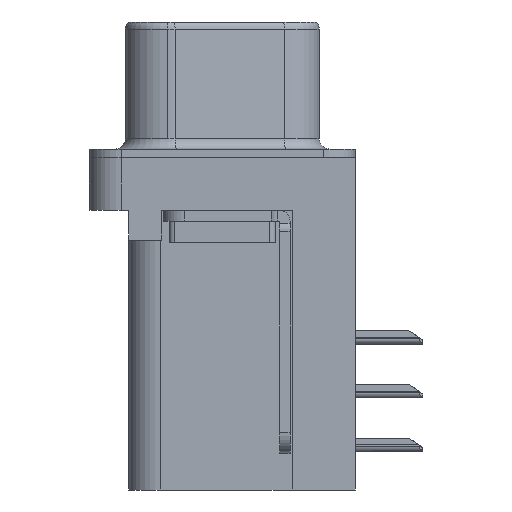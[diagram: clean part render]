
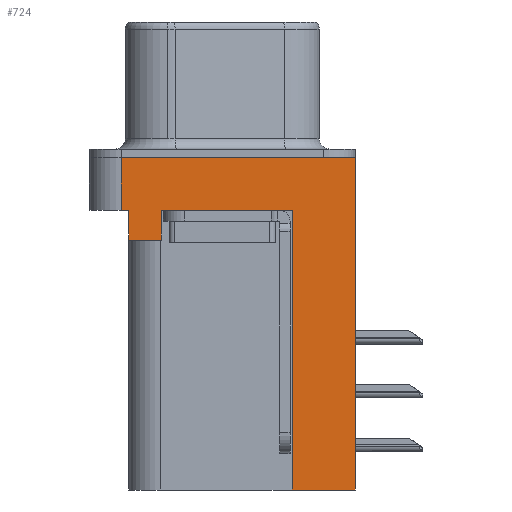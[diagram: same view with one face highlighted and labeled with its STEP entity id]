
A CAD part, left-side view. The second image highlights one B-rep face of the part: STEP entity #724.
In plain terms, the highlighted planar face has unit normal (-1, 0, 0).
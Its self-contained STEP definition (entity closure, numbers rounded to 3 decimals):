
#7 = LINE ( 'NONE', #4996, #25877 ) ;
#96 = VECTOR ( 'NONE', #20133, 1000. ) ;
#724 = ADVANCED_FACE ( 'NONE', ( #19348 ), #10806, .T. ) ;
#2074 = LINE ( 'NONE', #29223, #28957 ) ;
#3903 = CARTESIAN_POINT ( 'NONE',  ( -2.91, -6.275, 0. ) ) ;
#4432 = ORIENTED_EDGE ( 'NONE', *, *, #19202, .F. ) ;
#4996 = CARTESIAN_POINT ( 'NONE',  ( -2.91, -6.275, -2.5 ) ) ;
#5972 = EDGE_LOOP ( 'NONE', ( #6195, #30867, #8219, #24992, #11802, #33199, #10600, #34072, #4432, #23810 ) ) ;
#6113 = CARTESIAN_POINT ( 'NONE',  ( -2.91, -6.275, -2.5 ) ) ;
#6195 = ORIENTED_EDGE ( 'NONE', *, *, #15542, .F. ) ;
#6277 = LINE ( 'NONE', #28604, #28622 ) ;
#6493 = EDGE_CURVE ( 'NONE', #25158, #12339, #13691, .T. ) ;
#7218 = DIRECTION ( 'NONE',  ( 0., 1., 0. ) ) ;
#7662 = DIRECTION ( 'NONE',  ( 0., 0., 1. ) ) ;
#8219 = ORIENTED_EDGE ( 'NONE', *, *, #26451, .T. ) ;
#8778 = DIRECTION ( 'NONE',  ( 0., -1., 0. ) ) ;
#9291 = VERTEX_POINT ( 'NONE', #13595 ) ;
#9411 = CARTESIAN_POINT ( 'NONE',  ( -2.91, -3.295, -15.7 ) ) ;
#10600 = ORIENTED_EDGE ( 'NONE', *, *, #6493, .T. ) ;
#10667 = DIRECTION ( 'NONE',  ( 0., 0., 1. ) ) ;
#10806 = PLANE ( 'NONE',  #26622 ) ;
#10935 = VECTOR ( 'NONE', #10667, 1000. ) ;
#11802 = ORIENTED_EDGE ( 'NONE', *, *, #16735, .F. ) ;
#12339 = VERTEX_POINT ( 'NONE', #22976 ) ;
#12452 = DIRECTION ( 'NONE',  ( 0., 0., 1. ) ) ;
#12564 = DIRECTION ( 'NONE',  ( 0., 0., 1. ) ) ;
#12599 = CARTESIAN_POINT ( 'NONE',  ( -2.91, 2.895, -2.5 ) ) ;
#12738 = VERTEX_POINT ( 'NONE', #26831 ) ;
#13177 = VERTEX_POINT ( 'NONE', #34198 ) ;
#13595 = CARTESIAN_POINT ( 'NONE',  ( -2.91, 4.425, -2.5 ) ) ;
#13691 = LINE ( 'NONE', #6113, #27205 ) ;
#13717 = LINE ( 'NONE', #17897, #27230 ) ;
#13743 = CARTESIAN_POINT ( 'NONE',  ( -2.91, 4.775, -2.5 ) ) ;
#14590 = EDGE_CURVE ( 'NONE', #31923, #9291, #15024, .T. ) ;
#15024 = LINE ( 'NONE', #17603, #96 ) ;
#15542 = EDGE_CURVE ( 'NONE', #12738, #22639, #13717, .T. ) ;
#16201 = EDGE_CURVE ( 'NONE', #22479, #12738, #24565, .T. ) ;
#16735 = EDGE_CURVE ( 'NONE', #30396, #31923, #17400, .T. ) ;
#17128 = VECTOR ( 'NONE', #12452, 1000. ) ;
#17400 = LINE ( 'NONE', #25851, #31253 ) ;
#17603 = CARTESIAN_POINT ( 'NONE',  ( -2.91, 4.425, -3.9 ) ) ;
#17775 = CARTESIAN_POINT ( 'NONE',  ( -2.91, -3.295, -15.7 ) ) ;
#17841 = EDGE_CURVE ( 'NONE', #30396, #25158, #17972, .T. ) ;
#17897 = CARTESIAN_POINT ( 'NONE',  ( -2.91, -6.275, 0. ) ) ;
#17972 = LINE ( 'NONE', #29623, #10935 ) ;
#18573 = EDGE_CURVE ( 'NONE', #29237, #12339, #31879, .T. ) ;
#19202 = EDGE_CURVE ( 'NONE', #13177, #29237, #6277, .T. ) ;
#19348 = FACE_OUTER_BOUND ( 'NONE', #5972, .T. ) ;
#20133 = DIRECTION ( 'NONE',  ( 0., 0., 1. ) ) ;
#20556 = EDGE_CURVE ( 'NONE', #13177, #22639, #7, .T. ) ;
#20946 = DIRECTION ( 'NONE',  ( 0., 0., 1. ) ) ;
#21137 = CARTESIAN_POINT ( 'NONE',  ( -2.91, 4.425, -3.9 ) ) ;
#22404 = CARTESIAN_POINT ( 'NONE',  ( -2.91, 2.895, -3.9 ) ) ;
#22479 = VERTEX_POINT ( 'NONE', #13743 ) ;
#22639 = VERTEX_POINT ( 'NONE', #3903 ) ;
#22976 = CARTESIAN_POINT ( 'NONE',  ( -2.91, -3.295, -2.5 ) ) ;
#23595 = DIRECTION ( 'NONE',  ( 0., -1., 0. ) ) ;
#23810 = ORIENTED_EDGE ( 'NONE', *, *, #20556, .T. ) ;
#24565 = LINE ( 'NONE', #32193, #32220 ) ;
#24992 = ORIENTED_EDGE ( 'NONE', *, *, #14590, .F. ) ;
#25158 = VERTEX_POINT ( 'NONE', #12599 ) ;
#25851 = CARTESIAN_POINT ( 'NONE',  ( -2.91, 4.425, -3.9 ) ) ;
#25877 = VECTOR ( 'NONE', #7662, 1000. ) ;
#26451 = EDGE_CURVE ( 'NONE', #22479, #9291, #2074, .T. ) ;
#26622 = AXIS2_PLACEMENT_3D ( 'NONE', #34892, #35119, #12564 ) ;
#26831 = CARTESIAN_POINT ( 'NONE',  ( -2.91, 4.775, 0. ) ) ;
#27205 = VECTOR ( 'NONE', #8778, 1000. ) ;
#27230 = VECTOR ( 'NONE', #28903, 1000. ) ;
#28604 = CARTESIAN_POINT ( 'NONE',  ( -2.91, -3.295, -15.7 ) ) ;
#28622 = VECTOR ( 'NONE', #31583, 1000. ) ;
#28903 = DIRECTION ( 'NONE',  ( 0., -1., 0. ) ) ;
#28957 = VECTOR ( 'NONE', #23595, 1000. ) ;
#29223 = CARTESIAN_POINT ( 'NONE',  ( -2.91, -6.275, -2.5 ) ) ;
#29237 = VERTEX_POINT ( 'NONE', #9411 ) ;
#29623 = CARTESIAN_POINT ( 'NONE',  ( -2.91, 2.895, -3.9 ) ) ;
#30396 = VERTEX_POINT ( 'NONE', #22404 ) ;
#30867 = ORIENTED_EDGE ( 'NONE', *, *, #16201, .F. ) ;
#31253 = VECTOR ( 'NONE', #7218, 1000. ) ;
#31583 = DIRECTION ( 'NONE',  ( 0., 1., 0. ) ) ;
#31879 = LINE ( 'NONE', #17775, #17128 ) ;
#31923 = VERTEX_POINT ( 'NONE', #21137 ) ;
#32193 = CARTESIAN_POINT ( 'NONE',  ( -2.91, 4.775, -2.5 ) ) ;
#32220 = VECTOR ( 'NONE', #20946, 1000. ) ;
#33199 = ORIENTED_EDGE ( 'NONE', *, *, #17841, .T. ) ;
#34072 = ORIENTED_EDGE ( 'NONE', *, *, #18573, .F. ) ;
#34198 = CARTESIAN_POINT ( 'NONE',  ( -2.91, -6.275, -15.7 ) ) ;
#34892 = CARTESIAN_POINT ( 'NONE',  ( -2.91, -6.275, -2.5 ) ) ;
#35119 = DIRECTION ( 'NONE',  ( -1., 0., 0. ) ) ;
